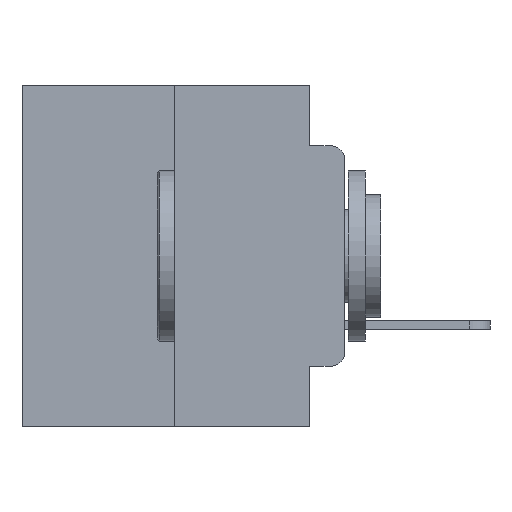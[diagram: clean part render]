
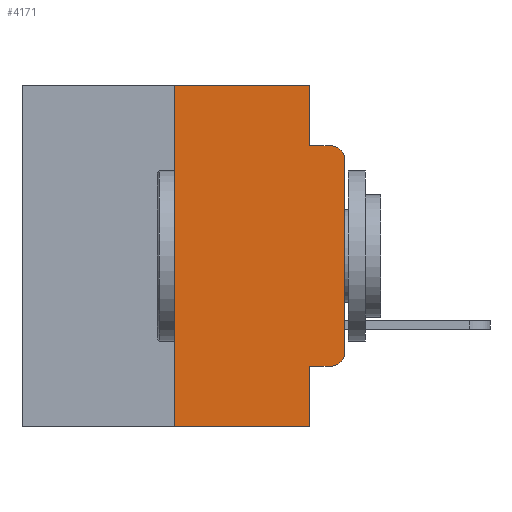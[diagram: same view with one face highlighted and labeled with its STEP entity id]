
A CAD part, left-side view. The second image highlights one B-rep face of the part: STEP entity #4171.
In plain terms, the highlighted planar face has unit normal (-1, 0, 0).
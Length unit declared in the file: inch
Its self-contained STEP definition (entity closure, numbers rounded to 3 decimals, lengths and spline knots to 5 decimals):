
#111 = ORIENTED_EDGE ( 'NONE', *, *, #17737, .F. ) ;
#168 = VERTEX_POINT ( 'NONE', #1886 ) ;
#1093 = EDGE_CURVE ( 'NONE', #168, #15299, #22506, .T. ) ;
#1449 = AXIS2_PLACEMENT_3D ( 'NONE', #14103, #11381, #9719 ) ;
#1548 = ORIENTED_EDGE ( 'NONE', *, *, #16622, .F. ) ;
#1559 = CARTESIAN_POINT ( 'NONE',  ( 0., 0.051, -0.0885 ) ) ;
#1565 = EDGE_CURVE ( 'NONE', #10905, #5749, #15658, .T. ) ;
#1886 = CARTESIAN_POINT ( 'NONE',  ( 0., 0., -0.1085 ) ) ;
#1994 = ORIENTED_EDGE ( 'NONE', *, *, #1565, .F. ) ;
#2057 = CARTESIAN_POINT ( 'NONE',  ( 0., 0.473, -0.5 ) ) ;
#2287 = DIRECTION ( 'NONE',  ( 0., -1., 0. ) ) ;
#2424 = AXIS2_PLACEMENT_3D ( 'NONE', #2827, #2793, #2684 ) ;
#2684 = DIRECTION ( 'NONE',  ( 0., 0., -1. ) ) ;
#2747 = ORIENTED_EDGE ( 'NONE', *, *, #6353, .T. ) ;
#2793 = DIRECTION ( 'NONE',  ( -1., 0., 0. ) ) ;
#2827 = CARTESIAN_POINT ( 'NONE',  ( 0., 0.02, -0.3915 ) ) ;
#3342 = AXIS2_PLACEMENT_3D ( 'NONE', #16363, #4922, #21231 ) ;
#3805 = DIRECTION ( 'NONE',  ( 0., 0., -1. ) ) ;
#3821 = DIRECTION ( 'NONE',  ( 0., 0., 1. ) ) ;
#3979 = DIRECTION ( 'NONE',  ( 0., -1., 0. ) ) ;
#4118 = VECTOR ( 'NONE', #3821, 39.37008 ) ;
#4171 = ADVANCED_FACE ( 'NONE', ( #10586 ), #22420, .F. ) ;
#4922 = DIRECTION ( 'NONE',  ( 1., 0., 0. ) ) ;
#5749 = VERTEX_POINT ( 'NONE', #21210 ) ;
#5905 = CARTESIAN_POINT ( 'NONE',  ( 0., 0., 0. ) ) ;
#6191 = CARTESIAN_POINT ( 'NONE',  ( 0., 0.25, -0.5 ) ) ;
#6353 = EDGE_CURVE ( 'NONE', #10905, #21618, #15836, .T. ) ;
#7208 = EDGE_CURVE ( 'NONE', #11299, #17840, #12189, .T. ) ;
#7778 = ORIENTED_EDGE ( 'NONE', *, *, #8150, .T. ) ;
#8150 = EDGE_CURVE ( 'NONE', #17840, #22688, #21222, .T. ) ;
#8250 = CARTESIAN_POINT ( 'NONE',  ( 0., 0.051, 0. ) ) ;
#9470 = VECTOR ( 'NONE', #3979, 39.37008 ) ;
#9568 = VECTOR ( 'NONE', #20740, 39.37008 ) ;
#9719 = DIRECTION ( 'NONE',  ( 0., 0., -1. ) ) ;
#10503 = ORIENTED_EDGE ( 'NONE', *, *, #7208, .T. ) ;
#10586 = FACE_OUTER_BOUND ( 'NONE', #23711, .T. ) ;
#10905 = VERTEX_POINT ( 'NONE', #6191 ) ;
#11299 = VERTEX_POINT ( 'NONE', #24608 ) ;
#11381 = DIRECTION ( 'NONE',  ( -1., 0., 0. ) ) ;
#11788 = ORIENTED_EDGE ( 'NONE', *, *, #12809, .F. ) ;
#12189 = LINE ( 'NONE', #25765, #22570 ) ;
#12342 = LINE ( 'NONE', #13540, #23348 ) ;
#12426 = ORIENTED_EDGE ( 'NONE', *, *, #21969, .T. ) ;
#12809 = EDGE_CURVE ( 'NONE', #14004, #19419, #12342, .T. ) ;
#12820 = LINE ( 'NONE', #8250, #15737 ) ;
#13308 = DIRECTION ( 'NONE',  ( 0., -1., 0. ) ) ;
#13540 = CARTESIAN_POINT ( 'NONE',  ( 0., 0.051, 0. ) ) ;
#13623 = DIRECTION ( 'NONE',  ( 0., 0., -1. ) ) ;
#14004 = VERTEX_POINT ( 'NONE', #20718 ) ;
#14103 = CARTESIAN_POINT ( 'NONE',  ( 0., 0.02, -0.1085 ) ) ;
#14574 = CARTESIAN_POINT ( 'NONE',  ( 0., 0.02, -0.0885 ) ) ;
#15096 = LINE ( 'NONE', #1559, #9470 ) ;
#15178 = VECTOR ( 'NONE', #2287, 39.37008 ) ;
#15299 = VERTEX_POINT ( 'NONE', #14574 ) ;
#15658 = LINE ( 'NONE', #27391, #4118 ) ;
#15737 = VECTOR ( 'NONE', #3805, 39.37008 ) ;
#15836 = LINE ( 'NONE', #2057, #15178 ) ;
#16363 = CARTESIAN_POINT ( 'NONE',  ( 0., 0.473, 0. ) ) ;
#16622 = EDGE_CURVE ( 'NONE', #19419, #15299, #15096, .T. ) ;
#17411 = LINE ( 'NONE', #27474, #26852 ) ;
#17737 = EDGE_CURVE ( 'NONE', #11299, #21618, #12820, .T. ) ;
#17840 = VERTEX_POINT ( 'NONE', #23245 ) ;
#19419 = VERTEX_POINT ( 'NONE', #20292 ) ;
#20057 = LINE ( 'NONE', #5905, #9568 ) ;
#20292 = CARTESIAN_POINT ( 'NONE',  ( 0., 0.051, -0.0885 ) ) ;
#20718 = CARTESIAN_POINT ( 'NONE',  ( 0., 0.051, 0. ) ) ;
#20740 = DIRECTION ( 'NONE',  ( 0., 0., 1. ) ) ;
#21210 = CARTESIAN_POINT ( 'NONE',  ( 0., 0.25, 0. ) ) ;
#21222 = CIRCLE ( 'NONE', #2424, 0.02 ) ;
#21231 = DIRECTION ( 'NONE',  ( 0., 0., -1. ) ) ;
#21618 = VERTEX_POINT ( 'NONE', #21890 ) ;
#21875 = ORIENTED_EDGE ( 'NONE', *, *, #24263, .F. ) ;
#21890 = CARTESIAN_POINT ( 'NONE',  ( 0., 0.051, -0.5 ) ) ;
#21969 = EDGE_CURVE ( 'NONE', #22688, #168, #20057, .T. ) ;
#22420 = PLANE ( 'NONE',  #3342 ) ;
#22488 = ORIENTED_EDGE ( 'NONE', *, *, #1093, .T. ) ;
#22506 = CIRCLE ( 'NONE', #1449, 0.02 ) ;
#22570 = VECTOR ( 'NONE', #25682, 39.37008 ) ;
#22688 = VERTEX_POINT ( 'NONE', #22770 ) ;
#22770 = CARTESIAN_POINT ( 'NONE',  ( 0., 0., -0.3915 ) ) ;
#23245 = CARTESIAN_POINT ( 'NONE',  ( 0., 0.02, -0.4115 ) ) ;
#23348 = VECTOR ( 'NONE', #13623, 39.37008 ) ;
#23711 = EDGE_LOOP ( 'NONE', ( #12426, #22488, #1548, #11788, #21875, #1994, #2747, #111, #10503, #7778 ) ) ;
#24263 = EDGE_CURVE ( 'NONE', #5749, #14004, #17411, .T. ) ;
#24608 = CARTESIAN_POINT ( 'NONE',  ( 0., 0.051, -0.4115 ) ) ;
#25682 = DIRECTION ( 'NONE',  ( 0., -1., 0. ) ) ;
#25765 = CARTESIAN_POINT ( 'NONE',  ( 0., 0.051, -0.4115 ) ) ;
#26852 = VECTOR ( 'NONE', #13308, 39.37008 ) ;
#27391 = CARTESIAN_POINT ( 'NONE',  ( 0., 0.25, 0. ) ) ;
#27474 = CARTESIAN_POINT ( 'NONE',  ( 0., 0.473, 0. ) ) ;
